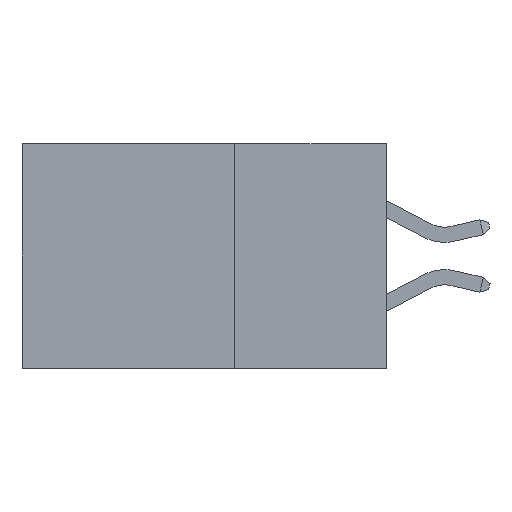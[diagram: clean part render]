
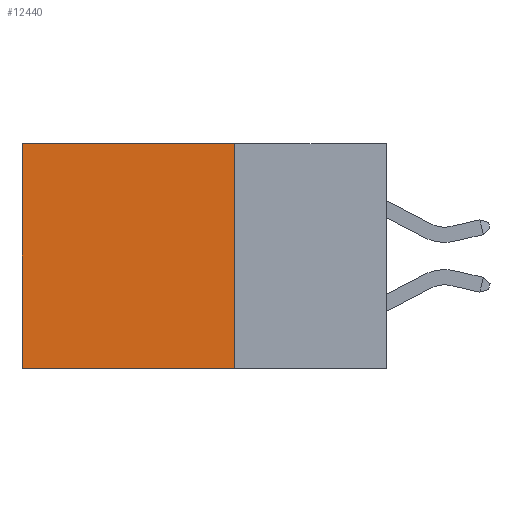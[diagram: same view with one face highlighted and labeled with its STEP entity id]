
A CAD part, left-side view. The second image highlights one B-rep face of the part: STEP entity #12440.
In plain terms, the highlighted planar face has unit normal (-1, 0, 0).
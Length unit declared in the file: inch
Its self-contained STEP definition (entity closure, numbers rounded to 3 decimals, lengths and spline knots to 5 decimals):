
#1881 = DIRECTION ( 'NONE',  ( 0., 1., 0. ) ) ;
#2716 = DIRECTION ( 'NONE',  ( 1., 0., 0. ) ) ;
#3033 = VECTOR ( 'NONE', #8565, 39.37008 ) ;
#4504 = PLANE ( 'NONE',  #14497 ) ;
#4875 = LINE ( 'NONE', #22870, #7982 ) ;
#5299 = EDGE_LOOP ( 'NONE', ( #9781, #15946, #18094, #22874 ) ) ;
#5390 = VECTOR ( 'NONE', #12900, 39.37008 ) ;
#5845 = VECTOR ( 'NONE', #1881, 39.37008 ) ;
#6177 = EDGE_CURVE ( 'NONE', #10435, #6286, #4875, .T. ) ;
#6286 = VERTEX_POINT ( 'NONE', #16323 ) ;
#6417 = LINE ( 'NONE', #21678, #5845 ) ;
#6525 = CARTESIAN_POINT ( 'NONE',  ( 0.298, 0.6, 0. ) ) ;
#7383 = LINE ( 'NONE', #12975, #5390 ) ;
#7982 = VECTOR ( 'NONE', #17238, 39.37008 ) ;
#8565 = DIRECTION ( 'NONE',  ( 0., 0., -1. ) ) ;
#9781 = ORIENTED_EDGE ( 'NONE', *, *, #15072, .T. ) ;
#10435 = VERTEX_POINT ( 'NONE', #12071 ) ;
#12071 = CARTESIAN_POINT ( 'NONE',  ( 0.298, 0.25, 0. ) ) ;
#12440 = ADVANCED_FACE ( 'NONE', ( #15831 ), #4504, .F. ) ;
#12900 = DIRECTION ( 'NONE',  ( 0., 1., 0. ) ) ;
#12975 = CARTESIAN_POINT ( 'NONE',  ( 0.298, 0.25, 0. ) ) ;
#14497 = AXIS2_PLACEMENT_3D ( 'NONE', #15301, #2716, #21039 ) ;
#14561 = VERTEX_POINT ( 'NONE', #6525 ) ;
#14793 = CARTESIAN_POINT ( 'NONE',  ( 0.298, 0.6, -0.37 ) ) ;
#15072 = EDGE_CURVE ( 'NONE', #14561, #22329, #19656, .T. ) ;
#15301 = CARTESIAN_POINT ( 'NONE',  ( 0.298, 0.25, 0. ) ) ;
#15831 = FACE_OUTER_BOUND ( 'NONE', #5299, .T. ) ;
#15946 = ORIENTED_EDGE ( 'NONE', *, *, #22959, .F. ) ;
#16323 = CARTESIAN_POINT ( 'NONE',  ( 0.298, 0.25, -0.37 ) ) ;
#17238 = DIRECTION ( 'NONE',  ( 0., 0., -1. ) ) ;
#18094 = ORIENTED_EDGE ( 'NONE', *, *, #6177, .F. ) ;
#19656 = LINE ( 'NONE', #21447, #3033 ) ;
#20940 = EDGE_CURVE ( 'NONE', #10435, #14561, #7383, .T. ) ;
#21039 = DIRECTION ( 'NONE',  ( 0., 0., -1. ) ) ;
#21447 = CARTESIAN_POINT ( 'NONE',  ( 0.298, 0.6, 0. ) ) ;
#21678 = CARTESIAN_POINT ( 'NONE',  ( 0.298, 0.25, -0.37 ) ) ;
#22329 = VERTEX_POINT ( 'NONE', #14793 ) ;
#22870 = CARTESIAN_POINT ( 'NONE',  ( 0.298, 0.25, 0. ) ) ;
#22874 = ORIENTED_EDGE ( 'NONE', *, *, #20940, .T. ) ;
#22959 = EDGE_CURVE ( 'NONE', #6286, #22329, #6417, .T. ) ;
